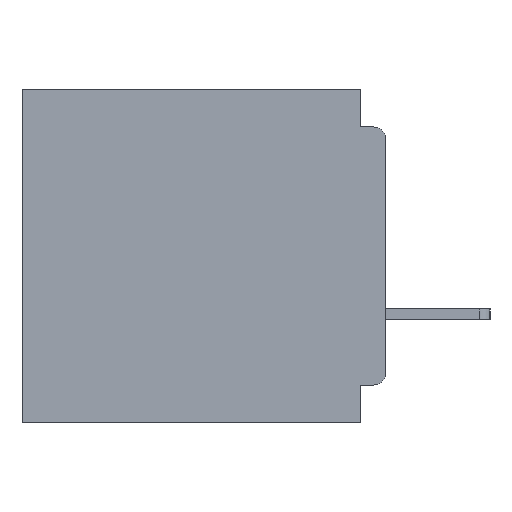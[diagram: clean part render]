
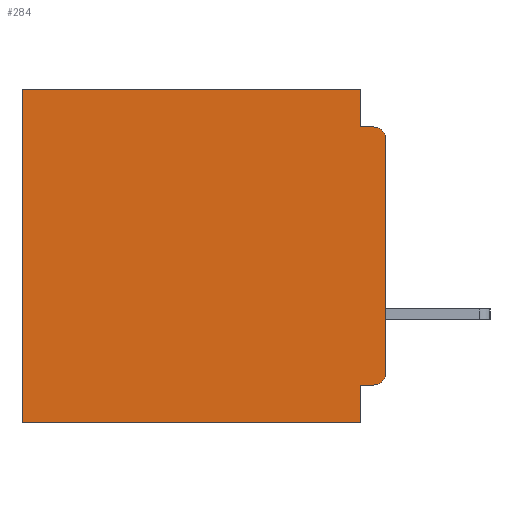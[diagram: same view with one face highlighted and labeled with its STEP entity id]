
A CAD part, left-side view. The second image highlights one B-rep face of the part: STEP entity #284.
In plain terms, the highlighted planar face has unit normal (-1, 0, 0).
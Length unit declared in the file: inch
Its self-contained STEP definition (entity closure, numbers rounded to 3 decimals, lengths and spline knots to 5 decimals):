
#130 = VERTEX_POINT ( 'NONE', #18108 ) ;
#172 = CARTESIAN_POINT ( 'NONE',  ( 0.3, 0., 0. ) ) ;
#188 = CARTESIAN_POINT ( 'NONE',  ( 0.3, 0., -0.06 ) ) ;
#284 = ADVANCED_FACE ( 'NONE', ( #1633 ), #566, .F. ) ;
#296 = CARTESIAN_POINT ( 'NONE',  ( 0.3, 0.015, -0.06 ) ) ;
#397 = EDGE_CURVE ( 'NONE', #21364, #3027, #4819, .T. ) ;
#409 = LINE ( 'NONE', #31069, #23587 ) ;
#566 = PLANE ( 'NONE',  #16689 ) ;
#1023 = VECTOR ( 'NONE', #13455, 39.37008 ) ;
#1143 = EDGE_CURVE ( 'NONE', #36885, #6280, #24756, .T. ) ;
#1180 = CARTESIAN_POINT ( 'NONE',  ( 0.3, 0.031, -0.045 ) ) ;
#1484 = CARTESIAN_POINT ( 'NONE',  ( 0.3, 0., -0.355 ) ) ;
#1633 = FACE_OUTER_BOUND ( 'NONE', #33415, .T. ) ;
#1839 = CARTESIAN_POINT ( 'NONE',  ( 0.3, 0.437, -0.4 ) ) ;
#1912 = LINE ( 'NONE', #1839, #1023 ) ;
#2318 = VERTEX_POINT ( 'NONE', #1180 ) ;
#2591 = VECTOR ( 'NONE', #4089, 39.37008 ) ;
#3027 = VERTEX_POINT ( 'NONE', #5400 ) ;
#3209 = DIRECTION ( 'NONE',  ( 0., 0., -1. ) ) ;
#3442 = AXIS2_PLACEMENT_3D ( 'NONE', #29236, #11966, #32149 ) ;
#4089 = DIRECTION ( 'NONE',  ( 0., 0., -1. ) ) ;
#4819 = LINE ( 'NONE', #20884, #19427 ) ;
#5400 = CARTESIAN_POINT ( 'NONE',  ( 0.3, 0., -0.34 ) ) ;
#5683 = CIRCLE ( 'NONE', #3442, 0.015 ) ;
#5994 = EDGE_CURVE ( 'NONE', #15986, #24944, #33068, .T. ) ;
#6280 = VERTEX_POINT ( 'NONE', #10788 ) ;
#6894 = CARTESIAN_POINT ( 'NONE',  ( 0.3, 0.031, -0.4 ) ) ;
#7080 = ORIENTED_EDGE ( 'NONE', *, *, #24225, .F. ) ;
#7529 = CARTESIAN_POINT ( 'NONE',  ( 0.3, 0.437, -0.4 ) ) ;
#7605 = VERTEX_POINT ( 'NONE', #10049 ) ;
#7941 = ORIENTED_EDGE ( 'NONE', *, *, #21374, .T. ) ;
#7951 = LINE ( 'NONE', #172, #31028 ) ;
#8883 = DIRECTION ( 'NONE',  ( 0., 1., 0. ) ) ;
#9308 = DIRECTION ( 'NONE',  ( 0., 1., 0. ) ) ;
#10049 = CARTESIAN_POINT ( 'NONE',  ( 0.3, 0.031, 0. ) ) ;
#10158 = LINE ( 'NONE', #6894, #26438 ) ;
#10363 = CARTESIAN_POINT ( 'NONE',  ( 0.3, 0., -0.4 ) ) ;
#10788 = CARTESIAN_POINT ( 'NONE',  ( 0.3, 0.031, -0.355 ) ) ;
#11086 = CARTESIAN_POINT ( 'NONE',  ( 0.3, 0.015, -0.045 ) ) ;
#11154 = ORIENTED_EDGE ( 'NONE', *, *, #36942, .T. ) ;
#11966 = DIRECTION ( 'NONE',  ( -1., 0., 0. ) ) ;
#12616 = EDGE_CURVE ( 'NONE', #7605, #130, #7951, .T. ) ;
#12971 = ORIENTED_EDGE ( 'NONE', *, *, #12616, .T. ) ;
#13455 = DIRECTION ( 'NONE',  ( 0., 0., -1. ) ) ;
#13849 = ORIENTED_EDGE ( 'NONE', *, *, #1143, .F. ) ;
#15986 = VERTEX_POINT ( 'NONE', #35291 ) ;
#16275 = CARTESIAN_POINT ( 'NONE',  ( 0.3, 0.015, -0.355 ) ) ;
#16510 = EDGE_CURVE ( 'NONE', #6280, #15986, #10158, .T. ) ;
#16689 = AXIS2_PLACEMENT_3D ( 'NONE', #33140, #32206, #35373 ) ;
#17097 = VECTOR ( 'NONE', #9308, 39.37008 ) ;
#17154 = DIRECTION ( 'NONE',  ( 0., 1., 0. ) ) ;
#18108 = CARTESIAN_POINT ( 'NONE',  ( 0.3, 0.437, 0. ) ) ;
#18538 = DIRECTION ( 'NONE',  ( 0., 0., -1. ) ) ;
#19427 = VECTOR ( 'NONE', #18538, 39.37008 ) ;
#20686 = DIRECTION ( 'NONE',  ( -1., 0., 0. ) ) ;
#20765 = AXIS2_PLACEMENT_3D ( 'NONE', #296, #20686, #3209 ) ;
#20884 = CARTESIAN_POINT ( 'NONE',  ( 0.3, 0., -0.4 ) ) ;
#21362 = VECTOR ( 'NONE', #17154, 39.37008 ) ;
#21364 = VERTEX_POINT ( 'NONE', #188 ) ;
#21374 = EDGE_CURVE ( 'NONE', #36885, #3027, #5683, .T. ) ;
#21625 = ORIENTED_EDGE ( 'NONE', *, *, #22565, .F. ) ;
#22565 = EDGE_CURVE ( 'NONE', #2318, #23207, #409, .T. ) ;
#23207 = VERTEX_POINT ( 'NONE', #11086 ) ;
#23587 = VECTOR ( 'NONE', #36990, 39.37008 ) ;
#24225 = EDGE_CURVE ( 'NONE', #7605, #2318, #32549, .T. ) ;
#24260 = DIRECTION ( 'NONE',  ( 0., 0., -1. ) ) ;
#24407 = CARTESIAN_POINT ( 'NONE',  ( 0.3, 0.031, 0. ) ) ;
#24756 = LINE ( 'NONE', #1484, #17097 ) ;
#24944 = VERTEX_POINT ( 'NONE', #7529 ) ;
#26438 = VECTOR ( 'NONE', #24260, 39.37008 ) ;
#28306 = ORIENTED_EDGE ( 'NONE', *, *, #5994, .F. ) ;
#29236 = CARTESIAN_POINT ( 'NONE',  ( 0.3, 0.015, -0.34 ) ) ;
#30108 = ORIENTED_EDGE ( 'NONE', *, *, #16510, .F. ) ;
#30595 = ORIENTED_EDGE ( 'NONE', *, *, #397, .F. ) ;
#31028 = VECTOR ( 'NONE', #8883, 39.37008 ) ;
#31069 = CARTESIAN_POINT ( 'NONE',  ( 0.3, 0., -0.045 ) ) ;
#32149 = DIRECTION ( 'NONE',  ( 0., 0., -1. ) ) ;
#32206 = DIRECTION ( 'NONE',  ( 1., 0., 0. ) ) ;
#32549 = LINE ( 'NONE', #24407, #2591 ) ;
#32954 = EDGE_CURVE ( 'NONE', #21364, #23207, #34127, .T. ) ;
#33068 = LINE ( 'NONE', #10363, #21362 ) ;
#33140 = CARTESIAN_POINT ( 'NONE',  ( 0.3, 0., -0.4 ) ) ;
#33415 = EDGE_LOOP ( 'NONE', ( #30595, #37052, #21625, #7080, #12971, #11154, #28306, #30108, #13849, #7941 ) ) ;
#34127 = CIRCLE ( 'NONE', #20765, 0.015 ) ;
#35291 = CARTESIAN_POINT ( 'NONE',  ( 0.3, 0.031, -0.4 ) ) ;
#35373 = DIRECTION ( 'NONE',  ( 0., 0., -1. ) ) ;
#36885 = VERTEX_POINT ( 'NONE', #16275 ) ;
#36942 = EDGE_CURVE ( 'NONE', #130, #24944, #1912, .T. ) ;
#36990 = DIRECTION ( 'NONE',  ( 0., -1., 0. ) ) ;
#37052 = ORIENTED_EDGE ( 'NONE', *, *, #32954, .T. ) ;
